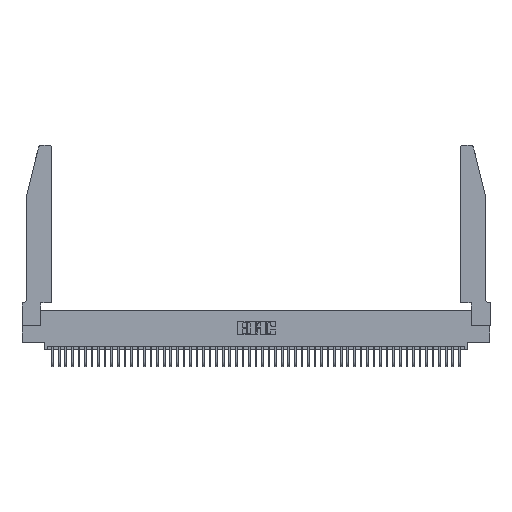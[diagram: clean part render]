
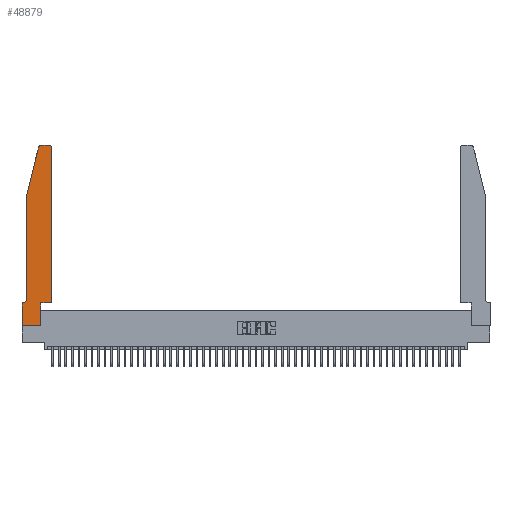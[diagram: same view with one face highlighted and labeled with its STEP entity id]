
A CAD part, top view. The second image highlights one B-rep face of the part: STEP entity #48879.
In plain terms, the highlighted planar face has unit normal (0, 0, 1).
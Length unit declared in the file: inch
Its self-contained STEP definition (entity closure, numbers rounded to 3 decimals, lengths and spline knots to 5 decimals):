
#240 = EDGE_CURVE ( 'NONE', #37900, #38900, #26891, .T. ) ;
#719 = CARTESIAN_POINT ( 'NONE',  ( 0.0755, 2., 0.37 ) ) ;
#2430 = CARTESIAN_POINT ( 'NONE',  ( 0.4505, 0.35, 0.37 ) ) ;
#3291 = CARTESIAN_POINT ( 'NONE',  ( 0.2605, 2.75, 0.37 ) ) ;
#4978 = DIRECTION ( 'NONE',  ( 0., -1., 0. ) ) ;
#5160 = EDGE_CURVE ( 'NONE', #35529, #13375, #25704, .T. ) ;
#5188 = EDGE_CURVE ( 'NONE', #26848, #15363, #35370, .T. ) ;
#6471 = VERTEX_POINT ( 'NONE', #50018 ) ;
#9490 = EDGE_CURVE ( 'NONE', #38900, #17743, #40413, .T. ) ;
#10722 = VECTOR ( 'NONE', #20981, 39.37008 ) ;
#11074 = CARTESIAN_POINT ( 'NONE',  ( 0.2865, 0., 0.37 ) ) ;
#12930 = CARTESIAN_POINT ( 'NONE',  ( 0.0755, 2., 0.37 ) ) ;
#13300 = CIRCLE ( 'NONE', #34838, 0.03 ) ;
#13375 = VERTEX_POINT ( 'NONE', #24255 ) ;
#13500 = DIRECTION ( 'NONE',  ( 0., 0., -1. ) ) ;
#13553 = EDGE_CURVE ( 'NONE', #34203, #26848, #37177, .T. ) ;
#15363 = VERTEX_POINT ( 'NONE', #40399 ) ;
#15378 = AXIS2_PLACEMENT_3D ( 'NONE', #38092, #13500, #42186 ) ;
#15549 = DIRECTION ( 'NONE',  ( 1., 0., 0. ) ) ;
#15672 = FACE_OUTER_BOUND ( 'NONE', #52175, .T. ) ;
#15951 = VECTOR ( 'NONE', #43422, 39.37008 ) ;
#16330 = ORIENTED_EDGE ( 'NONE', *, *, #47113, .T. ) ;
#16896 = ORIENTED_EDGE ( 'NONE', *, *, #5160, .T. ) ;
#17697 = ORIENTED_EDGE ( 'NONE', *, *, #18752, .T. ) ;
#17743 = VERTEX_POINT ( 'NONE', #2430 ) ;
#17776 = CARTESIAN_POINT ( 'NONE',  ( 0.4505, 0.35, 0.37 ) ) ;
#18752 = EDGE_CURVE ( 'NONE', #15363, #39641, #43071, .T. ) ;
#18857 = CARTESIAN_POINT ( 'NONE',  ( 0., 0.35, 0.37 ) ) ;
#18957 = LINE ( 'NONE', #27794, #49026 ) ;
#19063 = DIRECTION ( 'NONE',  ( 0., 0., 1. ) ) ;
#19217 = CARTESIAN_POINT ( 'NONE',  ( 0.284, 2.72, 0.37 ) ) ;
#19268 = EDGE_CURVE ( 'NONE', #37803, #34203, #27003, .T. ) ;
#20588 = EDGE_CURVE ( 'NONE', #48659, #37803, #40365, .T. ) ;
#20981 = DIRECTION ( 'NONE',  ( -1., 0., 0. ) ) ;
#22925 = LINE ( 'NONE', #37321, #10722 ) ;
#23333 = DIRECTION ( 'NONE',  ( 1., 0., 0. ) ) ;
#24255 = CARTESIAN_POINT ( 'NONE',  ( 0., 0., 0.37 ) ) ;
#24652 = DIRECTION ( 'NONE',  ( 1., 0., 0. ) ) ;
#25268 = DIRECTION ( 'NONE',  ( 0., -1., 0. ) ) ;
#25704 = LINE ( 'NONE', #33569, #28295 ) ;
#26372 = CARTESIAN_POINT ( 'NONE',  ( 0.0055, 0.35, 0.37 ) ) ;
#26848 = VERTEX_POINT ( 'NONE', #31364 ) ;
#26891 = LINE ( 'NONE', #47341, #15951 ) ;
#27003 = CIRCLE ( 'NONE', #47855, 0.03 ) ;
#27412 = CARTESIAN_POINT ( 'NONE',  ( 0.4205, 2.75, 0.37 ) ) ;
#27506 = ORIENTED_EDGE ( 'NONE', *, *, #34273, .T. ) ;
#27556 = VECTOR ( 'NONE', #41647, 39.37008 ) ;
#27794 = CARTESIAN_POINT ( 'NONE',  ( 0., 0., 0.37 ) ) ;
#28295 = VECTOR ( 'NONE', #25268, 39.37008 ) ;
#28639 = CARTESIAN_POINT ( 'NONE',  ( 0., 0.35, 0.37 ) ) ;
#29532 = EDGE_CURVE ( 'NONE', #6471, #48659, #13300, .T. ) ;
#30663 = ORIENTED_EDGE ( 'NONE', *, *, #240, .T. ) ;
#30692 = CARTESIAN_POINT ( 'NONE',  ( 0.284, 2.75, 0.37 ) ) ;
#30823 = VECTOR ( 'NONE', #42328, 39.37008 ) ;
#31364 = CARTESIAN_POINT ( 'NONE',  ( 0.0755, 2., 0.37 ) ) ;
#31571 = CARTESIAN_POINT ( 'NONE',  ( 0.25487, 2.72718, 0.37 ) ) ;
#32287 = ORIENTED_EDGE ( 'NONE', *, *, #20588, .T. ) ;
#32594 = VECTOR ( 'NONE', #41601, 39.37008 ) ;
#33213 = CARTESIAN_POINT ( 'NONE',  ( 0.4505, 0.35, 0.37 ) ) ;
#33569 = CARTESIAN_POINT ( 'NONE',  ( 0., 0., 0.37 ) ) ;
#34094 = VECTOR ( 'NONE', #4978, 39.37008 ) ;
#34203 = VERTEX_POINT ( 'NONE', #31571 ) ;
#34273 = EDGE_CURVE ( 'NONE', #13375, #37900, #18957, .T. ) ;
#34838 = AXIS2_PLACEMENT_3D ( 'NONE', #43616, #19063, #47686 ) ;
#35370 = LINE ( 'NONE', #719, #34094 ) ;
#35481 = ORIENTED_EDGE ( 'NONE', *, *, #9490, .T. ) ;
#35529 = VERTEX_POINT ( 'NONE', #18857 ) ;
#36185 = DIRECTION ( 'NONE',  ( -1., 0., 0. ) ) ;
#37177 = LINE ( 'NONE', #12930, #27556 ) ;
#37321 = CARTESIAN_POINT ( 'NONE',  ( 0.0755, 0.35, 0.37 ) ) ;
#37803 = VERTEX_POINT ( 'NONE', #30692 ) ;
#37900 = VERTEX_POINT ( 'NONE', #11074 ) ;
#38092 = CARTESIAN_POINT ( 'NONE',  ( 0.0055, 0.42, 0.37 ) ) ;
#38900 = VERTEX_POINT ( 'NONE', #50922 ) ;
#39183 = ORIENTED_EDGE ( 'NONE', *, *, #5188, .T. ) ;
#39641 = VERTEX_POINT ( 'NONE', #26372 ) ;
#40365 = LINE ( 'NONE', #3291, #52444 ) ;
#40399 = CARTESIAN_POINT ( 'NONE',  ( 0.0755, 0.42, 0.37 ) ) ;
#40413 = LINE ( 'NONE', #17776, #30823 ) ;
#40968 = ORIENTED_EDGE ( 'NONE', *, *, #19268, .T. ) ;
#41601 = DIRECTION ( 'NONE',  ( 0., 1., 0. ) ) ;
#41647 = DIRECTION ( 'NONE',  ( -0.239, -0.971, 0. ) ) ;
#42186 = DIRECTION ( 'NONE',  ( -1., 0., 0. ) ) ;
#42328 = DIRECTION ( 'NONE',  ( 1., 0., 0. ) ) ;
#42570 = AXIS2_PLACEMENT_3D ( 'NONE', #28639, #49155, #24652 ) ;
#43071 = CIRCLE ( 'NONE', #15378, 0.07 ) ;
#43422 = DIRECTION ( 'NONE',  ( 0., 1., 0. ) ) ;
#43616 = CARTESIAN_POINT ( 'NONE',  ( 0.4205, 2.72, 0.37 ) ) ;
#45047 = ORIENTED_EDGE ( 'NONE', *, *, #13553, .T. ) ;
#45076 = PLANE ( 'NONE',  #42570 ) ;
#47095 = EDGE_CURVE ( 'NONE', #39641, #35529, #22925, .T. ) ;
#47113 = EDGE_CURVE ( 'NONE', #17743, #6471, #52950, .T. ) ;
#47341 = CARTESIAN_POINT ( 'NONE',  ( 0.2865, 0.35, 0.37 ) ) ;
#47686 = DIRECTION ( 'NONE',  ( 1., 0., 0. ) ) ;
#47850 = DIRECTION ( 'NONE',  ( 0., 0., 1. ) ) ;
#47855 = AXIS2_PLACEMENT_3D ( 'NONE', #19217, #47850, #23333 ) ;
#48659 = VERTEX_POINT ( 'NONE', #27412 ) ;
#48879 = ADVANCED_FACE ( 'NONE', ( #15672 ), #45076, .T. ) ;
#49026 = VECTOR ( 'NONE', #15549, 39.37008 ) ;
#49107 = ORIENTED_EDGE ( 'NONE', *, *, #29532, .T. ) ;
#49155 = DIRECTION ( 'NONE',  ( 0., 0., 1. ) ) ;
#50018 = CARTESIAN_POINT ( 'NONE',  ( 0.4505, 2.72, 0.37 ) ) ;
#50871 = ORIENTED_EDGE ( 'NONE', *, *, #47095, .T. ) ;
#50922 = CARTESIAN_POINT ( 'NONE',  ( 0.2865, 0.35, 0.37 ) ) ;
#52175 = EDGE_LOOP ( 'NONE', ( #32287, #40968, #45047, #39183, #17697, #50871, #16896, #27506, #30663, #35481, #16330, #49107 ) ) ;
#52444 = VECTOR ( 'NONE', #36185, 39.37008 ) ;
#52950 = LINE ( 'NONE', #33213, #32594 ) ;
